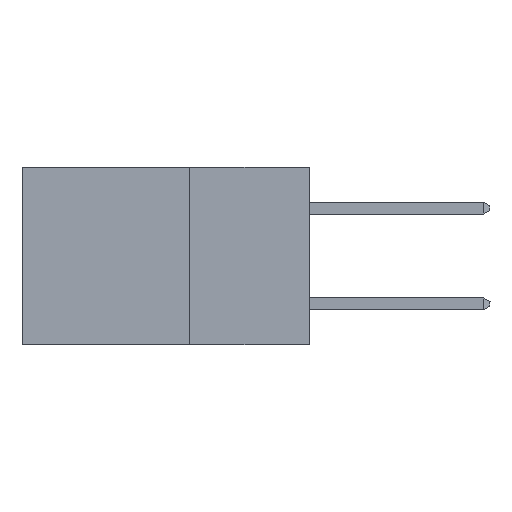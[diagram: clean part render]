
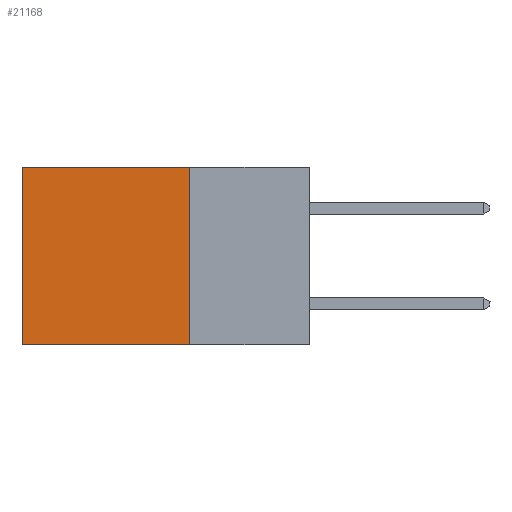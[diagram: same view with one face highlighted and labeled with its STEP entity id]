
A CAD part, left-side view. The second image highlights one B-rep face of the part: STEP entity #21168.
In plain terms, the highlighted planar face has unit normal (-1, 0, 0).
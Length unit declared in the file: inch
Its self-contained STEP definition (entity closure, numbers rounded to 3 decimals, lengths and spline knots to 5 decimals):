
#724 = CARTESIAN_POINT ( 'NONE',  ( 0.2875, 0.25, 0. ) ) ;
#729 = LINE ( 'NONE', #34231, #20552 ) ;
#3455 = LINE ( 'NONE', #14099, #32951 ) ;
#3566 = ORIENTED_EDGE ( 'NONE', *, *, #40530, .F. ) ;
#4272 = DIRECTION ( 'NONE',  ( 0., 1., 0. ) ) ;
#4700 = CARTESIAN_POINT ( 'NONE',  ( 0.2875, 0.25, 0. ) ) ;
#9439 = DIRECTION ( 'NONE',  ( 0., 0., -1. ) ) ;
#10095 = DIRECTION ( 'NONE',  ( 0., 0., -1. ) ) ;
#10766 = CARTESIAN_POINT ( 'NONE',  ( 0.2875, 0.6, -0.37 ) ) ;
#11133 = EDGE_CURVE ( 'NONE', #11830, #30997, #22542, .T. ) ;
#11830 = VERTEX_POINT ( 'NONE', #34648 ) ;
#12647 = AXIS2_PLACEMENT_3D ( 'NONE', #32920, #20294, #10095 ) ;
#14099 = CARTESIAN_POINT ( 'NONE',  ( 0.2875, 0.25, 0. ) ) ;
#18924 = ORIENTED_EDGE ( 'NONE', *, *, #31365, .T. ) ;
#18977 = FACE_OUTER_BOUND ( 'NONE', #39482, .T. ) ;
#19413 = PLANE ( 'NONE',  #12647 ) ;
#20294 = DIRECTION ( 'NONE',  ( 1., 0., 0. ) ) ;
#20335 = ORIENTED_EDGE ( 'NONE', *, *, #11133, .T. ) ;
#20552 = VECTOR ( 'NONE', #4272, 39.37008 ) ;
#21168 = ADVANCED_FACE ( 'NONE', ( #18977 ), #19413, .F. ) ;
#21369 = LINE ( 'NONE', #724, #21906 ) ;
#21906 = VECTOR ( 'NONE', #37773, 39.37008 ) ;
#22542 = LINE ( 'NONE', #26077, #32414 ) ;
#22790 = VERTEX_POINT ( 'NONE', #38901 ) ;
#26077 = CARTESIAN_POINT ( 'NONE',  ( 0.2875, 0.6, 0. ) ) ;
#30979 = ORIENTED_EDGE ( 'NONE', *, *, #32797, .F. ) ;
#30997 = VERTEX_POINT ( 'NONE', #10766 ) ;
#31365 = EDGE_CURVE ( 'NONE', #31436, #11830, #21369, .T. ) ;
#31436 = VERTEX_POINT ( 'NONE', #4700 ) ;
#32414 = VECTOR ( 'NONE', #9439, 39.37008 ) ;
#32797 = EDGE_CURVE ( 'NONE', #22790, #30997, #729, .T. ) ;
#32920 = CARTESIAN_POINT ( 'NONE',  ( 0.2875, 0.25, 0. ) ) ;
#32951 = VECTOR ( 'NONE', #40931, 39.37008 ) ;
#34231 = CARTESIAN_POINT ( 'NONE',  ( 0.2875, 0.25, -0.37 ) ) ;
#34648 = CARTESIAN_POINT ( 'NONE',  ( 0.2875, 0.6, 0. ) ) ;
#37773 = DIRECTION ( 'NONE',  ( 0., 1., 0. ) ) ;
#38901 = CARTESIAN_POINT ( 'NONE',  ( 0.2875, 0.25, -0.37 ) ) ;
#39482 = EDGE_LOOP ( 'NONE', ( #20335, #30979, #3566, #18924 ) ) ;
#40530 = EDGE_CURVE ( 'NONE', #31436, #22790, #3455, .T. ) ;
#40931 = DIRECTION ( 'NONE',  ( 0., 0., -1. ) ) ;
